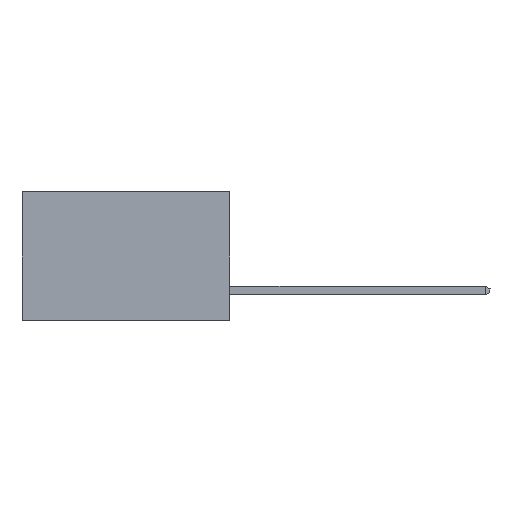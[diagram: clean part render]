
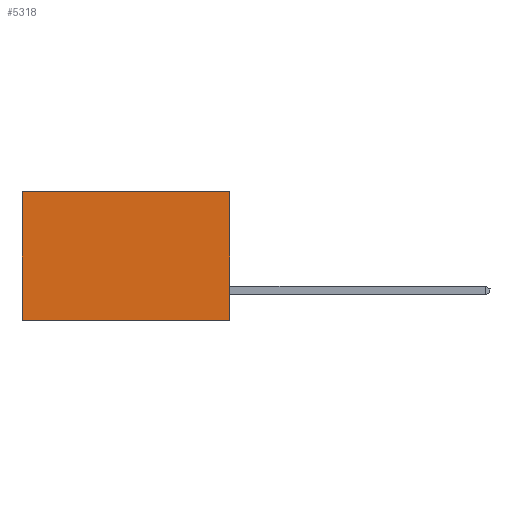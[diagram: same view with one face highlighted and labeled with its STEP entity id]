
A CAD part, left-side view. The second image highlights one B-rep face of the part: STEP entity #5318.
In plain terms, the highlighted planar face has unit normal (-1, 0, 0).
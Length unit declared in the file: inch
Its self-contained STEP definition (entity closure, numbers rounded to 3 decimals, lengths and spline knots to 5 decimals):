
#699 = LINE ( 'NONE', #2567, #9384 ) ;
#1405 = EDGE_CURVE ( 'NONE', #1568, #9127, #699, .T. ) ;
#1568 = VERTEX_POINT ( 'NONE', #3966 ) ;
#2567 = CARTESIAN_POINT ( 'NONE',  ( 0.2615, 0., -0.37 ) ) ;
#3168 = CARTESIAN_POINT ( 'NONE',  ( 0.2615, 0., 0. ) ) ;
#3358 = VECTOR ( 'NONE', #9243, 39.37008 ) ;
#3570 = CARTESIAN_POINT ( 'NONE',  ( 0.2615, 0.6, -0.37 ) ) ;
#3592 = DIRECTION ( 'NONE',  ( 0., 1., 0. ) ) ;
#3611 = DIRECTION ( 'NONE',  ( 0., 0., -1. ) ) ;
#3667 = LINE ( 'NONE', #5333, #3358 ) ;
#3840 = LINE ( 'NONE', #6767, #11528 ) ;
#3966 = CARTESIAN_POINT ( 'NONE',  ( 0.2615, 0., -0.37 ) ) ;
#4111 = CARTESIAN_POINT ( 'NONE',  ( 0.2615, 0., 0. ) ) ;
#4696 = EDGE_LOOP ( 'NONE', ( #5693, #10433, #7992, #9266 ) ) ;
#5318 = ADVANCED_FACE ( 'NONE', ( #10411 ), #9438, .F. ) ;
#5333 = CARTESIAN_POINT ( 'NONE',  ( 0.2615, 0.6, -0.37 ) ) ;
#5693 = ORIENTED_EDGE ( 'NONE', *, *, #9780, .T. ) ;
#5805 = DIRECTION ( 'NONE',  ( 0., 0., -1. ) ) ;
#6767 = CARTESIAN_POINT ( 'NONE',  ( 0.2615, 0., -0.37 ) ) ;
#7992 = ORIENTED_EDGE ( 'NONE', *, *, #8793, .F. ) ;
#8078 = DIRECTION ( 'NONE',  ( 0., 1., 0. ) ) ;
#8248 = VECTOR ( 'NONE', #8078, 39.37008 ) ;
#8463 = CARTESIAN_POINT ( 'NONE',  ( 0.2615, 0., -0.37 ) ) ;
#8793 = EDGE_CURVE ( 'NONE', #12559, #1568, #3840, .T. ) ;
#9127 = VERTEX_POINT ( 'NONE', #3570 ) ;
#9205 = VERTEX_POINT ( 'NONE', #10873 ) ;
#9243 = DIRECTION ( 'NONE',  ( 0., 0., -1. ) ) ;
#9266 = ORIENTED_EDGE ( 'NONE', *, *, #11328, .T. ) ;
#9384 = VECTOR ( 'NONE', #3592, 39.37008 ) ;
#9438 = PLANE ( 'NONE',  #10310 ) ;
#9780 = EDGE_CURVE ( 'NONE', #9205, #9127, #3667, .T. ) ;
#10147 = LINE ( 'NONE', #4111, #8248 ) ;
#10310 = AXIS2_PLACEMENT_3D ( 'NONE', #8463, #12415, #3611 ) ;
#10411 = FACE_OUTER_BOUND ( 'NONE', #4696, .T. ) ;
#10433 = ORIENTED_EDGE ( 'NONE', *, *, #1405, .F. ) ;
#10873 = CARTESIAN_POINT ( 'NONE',  ( 0.2615, 0.6, 0. ) ) ;
#11328 = EDGE_CURVE ( 'NONE', #12559, #9205, #10147, .T. ) ;
#11528 = VECTOR ( 'NONE', #5805, 39.37008 ) ;
#12415 = DIRECTION ( 'NONE',  ( 1., 0., 0. ) ) ;
#12559 = VERTEX_POINT ( 'NONE', #3168 ) ;
